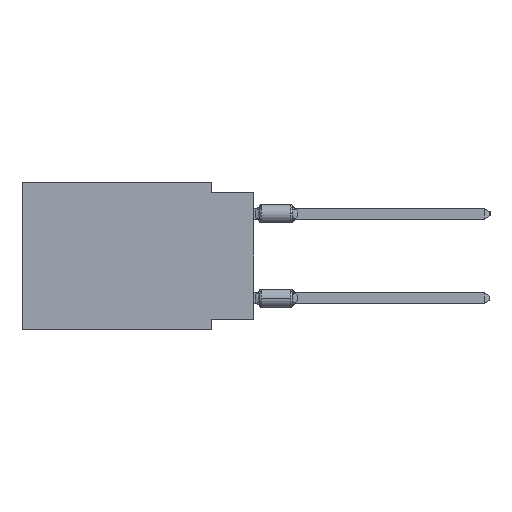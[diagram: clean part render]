
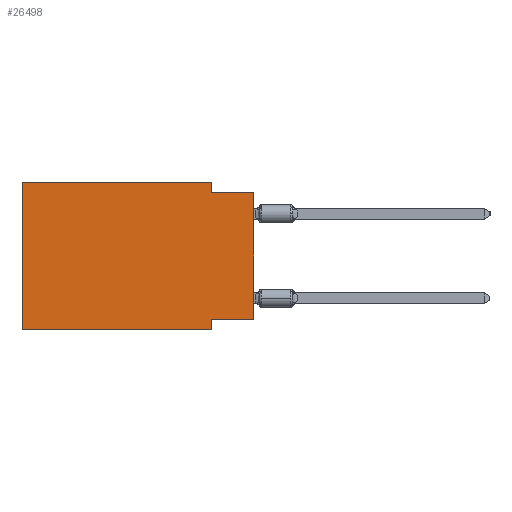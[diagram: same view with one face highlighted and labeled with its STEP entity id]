
A CAD part, left-side view. The second image highlights one B-rep face of the part: STEP entity #26498.
In plain terms, the highlighted planar face has unit normal (-1, 0, 0).
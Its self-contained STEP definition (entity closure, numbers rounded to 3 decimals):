
#793 = CARTESIAN_POINT ( 'NONE',  ( 0., 0., -8.255 ) ) ;
#1601 = ORIENTED_EDGE ( 'NONE', *, *, #28045, .T. ) ;
#1947 = DIRECTION ( 'NONE',  ( 0., 0., -1. ) ) ;
#2144 = CARTESIAN_POINT ( 'NONE',  ( 0., 2.54, -0.635 ) ) ;
#2154 = VERTEX_POINT ( 'NONE', #19513 ) ;
#4233 = CARTESIAN_POINT ( 'NONE',  ( 0., 0., -0.635 ) ) ;
#4989 = CARTESIAN_POINT ( 'NONE',  ( 0., 13.97, -8.89 ) ) ;
#5880 = VERTEX_POINT ( 'NONE', #4989 ) ;
#6050 = ORIENTED_EDGE ( 'NONE', *, *, #11606, .T. ) ;
#6443 = ORIENTED_EDGE ( 'NONE', *, *, #23575, .F. ) ;
#7020 = VERTEX_POINT ( 'NONE', #26485 ) ;
#7474 = EDGE_CURVE ( 'NONE', #5880, #2154, #26968, .T. ) ;
#7980 = VERTEX_POINT ( 'NONE', #26926 ) ;
#8830 = CARTESIAN_POINT ( 'NONE',  ( 0., 2.54, -8.89 ) ) ;
#8943 = LINE ( 'NONE', #4233, #27745 ) ;
#9323 = CARTESIAN_POINT ( 'NONE',  ( 0., 13.97, 0. ) ) ;
#9805 = VECTOR ( 'NONE', #28363, 1000. ) ;
#10279 = EDGE_LOOP ( 'NONE', ( #6050, #34767, #11530, #22959, #19067, #1601, #36482, #6443 ) ) ;
#11406 = VECTOR ( 'NONE', #30093, 1000. ) ;
#11530 = ORIENTED_EDGE ( 'NONE', *, *, #26048, .F. ) ;
#11606 = EDGE_CURVE ( 'NONE', #12470, #7020, #16877, .T. ) ;
#12470 = VERTEX_POINT ( 'NONE', #793 ) ;
#13420 = VECTOR ( 'NONE', #20170, 1000. ) ;
#16192 = VECTOR ( 'NONE', #20933, 1000. ) ;
#16306 = VECTOR ( 'NONE', #30510, 1000. ) ;
#16867 = LINE ( 'NONE', #22458, #9805 ) ;
#16877 = LINE ( 'NONE', #36500, #35322 ) ;
#18670 = PLANE ( 'NONE',  #21011 ) ;
#19067 = ORIENTED_EDGE ( 'NONE', *, *, #7474, .F. ) ;
#19513 = CARTESIAN_POINT ( 'NONE',  ( 0., 13.97, 0. ) ) ;
#19982 = LINE ( 'NONE', #8830, #13420 ) ;
#20138 = VERTEX_POINT ( 'NONE', #27238 ) ;
#20170 = DIRECTION ( 'NONE',  ( 0., 0., -1. ) ) ;
#20933 = DIRECTION ( 'NONE',  ( 0., -1., 0. ) ) ;
#21011 = AXIS2_PLACEMENT_3D ( 'NONE', #24420, #35514, #1947 ) ;
#22138 = LINE ( 'NONE', #28239, #26875 ) ;
#22458 = CARTESIAN_POINT ( 'NONE',  ( 0., 0., -8.255 ) ) ;
#22809 = EDGE_CURVE ( 'NONE', #2154, #7980, #34702, .T. ) ;
#22959 = ORIENTED_EDGE ( 'NONE', *, *, #22809, .F. ) ;
#23575 = EDGE_CURVE ( 'NONE', #12470, #32213, #16867, .T. ) ;
#23826 = VERTEX_POINT ( 'NONE', #2144 ) ;
#23918 = DIRECTION ( 'NONE',  ( 0., -1., 0. ) ) ;
#24056 = EDGE_CURVE ( 'NONE', #32213, #20138, #19982, .T. ) ;
#24420 = CARTESIAN_POINT ( 'NONE',  ( 0., 13.97, 0. ) ) ;
#26048 = EDGE_CURVE ( 'NONE', #7980, #23826, #22138, .T. ) ;
#26485 = CARTESIAN_POINT ( 'NONE',  ( 0., 0., -0.635 ) ) ;
#26498 = ADVANCED_FACE ( 'NONE', ( #27565 ), #18670, .F. ) ;
#26669 = LINE ( 'NONE', #29608, #16192 ) ;
#26875 = VECTOR ( 'NONE', #27882, 1000. ) ;
#26926 = CARTESIAN_POINT ( 'NONE',  ( 0., 2.54, 0. ) ) ;
#26968 = LINE ( 'NONE', #33048, #11406 ) ;
#27238 = CARTESIAN_POINT ( 'NONE',  ( 0., 2.54, -8.89 ) ) ;
#27565 = FACE_OUTER_BOUND ( 'NONE', #10279, .T. ) ;
#27745 = VECTOR ( 'NONE', #23918, 1000. ) ;
#27882 = DIRECTION ( 'NONE',  ( 0., 0., -1. ) ) ;
#28045 = EDGE_CURVE ( 'NONE', #5880, #20138, #26669, .T. ) ;
#28239 = CARTESIAN_POINT ( 'NONE',  ( 0., 2.54, 0. ) ) ;
#28363 = DIRECTION ( 'NONE',  ( 0., 1., 0. ) ) ;
#29608 = CARTESIAN_POINT ( 'NONE',  ( 0., 13.97, -8.89 ) ) ;
#30093 = DIRECTION ( 'NONE',  ( 0., 0., 1. ) ) ;
#30510 = DIRECTION ( 'NONE',  ( 0., -1., 0. ) ) ;
#32002 = EDGE_CURVE ( 'NONE', #23826, #7020, #8943, .T. ) ;
#32213 = VERTEX_POINT ( 'NONE', #33498 ) ;
#33048 = CARTESIAN_POINT ( 'NONE',  ( 0., 13.97, 0. ) ) ;
#33498 = CARTESIAN_POINT ( 'NONE',  ( 0., 2.54, -8.255 ) ) ;
#33893 = DIRECTION ( 'NONE',  ( 0., 0., 1. ) ) ;
#34702 = LINE ( 'NONE', #9323, #16306 ) ;
#34767 = ORIENTED_EDGE ( 'NONE', *, *, #32002, .F. ) ;
#35322 = VECTOR ( 'NONE', #33893, 1000. ) ;
#35514 = DIRECTION ( 'NONE',  ( 1., 0., 0. ) ) ;
#36482 = ORIENTED_EDGE ( 'NONE', *, *, #24056, .F. ) ;
#36500 = CARTESIAN_POINT ( 'NONE',  ( 0., 0., 0. ) ) ;
